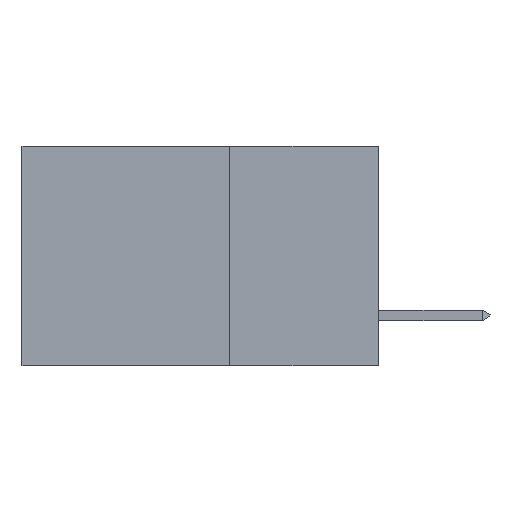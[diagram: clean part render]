
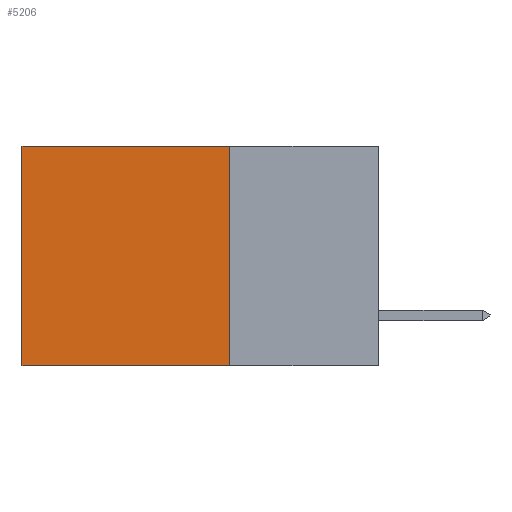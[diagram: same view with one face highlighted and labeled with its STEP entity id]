
A CAD part, left-side view. The second image highlights one B-rep face of the part: STEP entity #5206.
In plain terms, the highlighted planar face has unit normal (-1, 0, 0).
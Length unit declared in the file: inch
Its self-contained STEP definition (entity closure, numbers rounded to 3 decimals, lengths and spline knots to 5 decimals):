
#109 = ORIENTED_EDGE ( 'NONE', *, *, #8144, .F. ) ;
#133 = CARTESIAN_POINT ( 'NONE',  ( 0.2615, 0.25, -0.37 ) ) ;
#196 = DIRECTION ( 'NONE',  ( 0., 1., 0. ) ) ;
#473 = DIRECTION ( 'NONE',  ( 1., 0., 0. ) ) ;
#1700 = LINE ( 'NONE', #133, #12515 ) ;
#1868 = LINE ( 'NONE', #12715, #5414 ) ;
#2249 = CARTESIAN_POINT ( 'NONE',  ( 0.2615, 0.6, -0.37 ) ) ;
#3829 = DIRECTION ( 'NONE',  ( 0., 0., -1. ) ) ;
#3994 = CARTESIAN_POINT ( 'NONE',  ( 0.2615, 0.25, -0.37 ) ) ;
#4366 = CARTESIAN_POINT ( 'NONE',  ( 0.2615, 0.25, 0. ) ) ;
#5109 = DIRECTION ( 'NONE',  ( 0., 0., -1. ) ) ;
#5151 = ORIENTED_EDGE ( 'NONE', *, *, #9462, .T. ) ;
#5206 = ADVANCED_FACE ( 'NONE', ( #6182 ), #12075, .F. ) ;
#5414 = VECTOR ( 'NONE', #196, 39.37008 ) ;
#5934 = EDGE_LOOP ( 'NONE', ( #5151, #17600, #109, #14197 ) ) ;
#6182 = FACE_OUTER_BOUND ( 'NONE', #5934, .T. ) ;
#7778 = EDGE_CURVE ( 'NONE', #15948, #9743, #1868, .T. ) ;
#8144 = EDGE_CURVE ( 'NONE', #15948, #15203, #13882, .T. ) ;
#9462 = EDGE_CURVE ( 'NONE', #9743, #15604, #10822, .T. ) ;
#9743 = VERTEX_POINT ( 'NONE', #17434 ) ;
#10510 = AXIS2_PLACEMENT_3D ( 'NONE', #17608, #473, #5109 ) ;
#10820 = EDGE_CURVE ( 'NONE', #15203, #15604, #1700, .T. ) ;
#10822 = LINE ( 'NONE', #2249, #11798 ) ;
#11798 = VECTOR ( 'NONE', #3829, 39.37008 ) ;
#12075 = PLANE ( 'NONE',  #10510 ) ;
#12515 = VECTOR ( 'NONE', #16909, 39.37008 ) ;
#12715 = CARTESIAN_POINT ( 'NONE',  ( 0.2615, 0.25, 0. ) ) ;
#13882 = LINE ( 'NONE', #3994, #16541 ) ;
#14197 = ORIENTED_EDGE ( 'NONE', *, *, #7778, .T. ) ;
#15203 = VERTEX_POINT ( 'NONE', #16829 ) ;
#15545 = CARTESIAN_POINT ( 'NONE',  ( 0.2615, 0.6, -0.37 ) ) ;
#15604 = VERTEX_POINT ( 'NONE', #15545 ) ;
#15948 = VERTEX_POINT ( 'NONE', #4366 ) ;
#16519 = DIRECTION ( 'NONE',  ( 0., 0., -1. ) ) ;
#16541 = VECTOR ( 'NONE', #16519, 39.37008 ) ;
#16829 = CARTESIAN_POINT ( 'NONE',  ( 0.2615, 0.25, -0.37 ) ) ;
#16909 = DIRECTION ( 'NONE',  ( 0., 1., 0. ) ) ;
#17434 = CARTESIAN_POINT ( 'NONE',  ( 0.2615, 0.6, 0. ) ) ;
#17600 = ORIENTED_EDGE ( 'NONE', *, *, #10820, .F. ) ;
#17608 = CARTESIAN_POINT ( 'NONE',  ( 0.2615, 0.25, -0.37 ) ) ;
